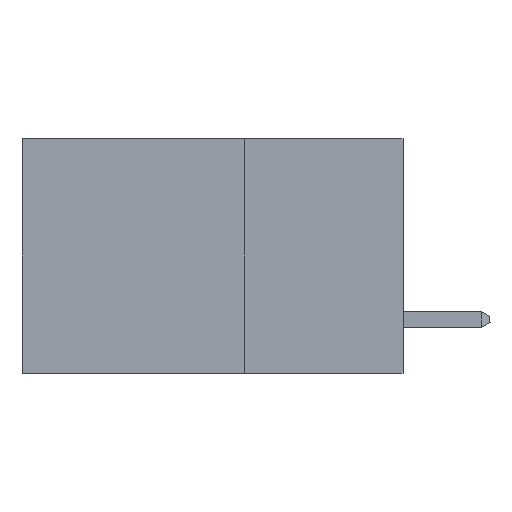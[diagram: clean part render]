
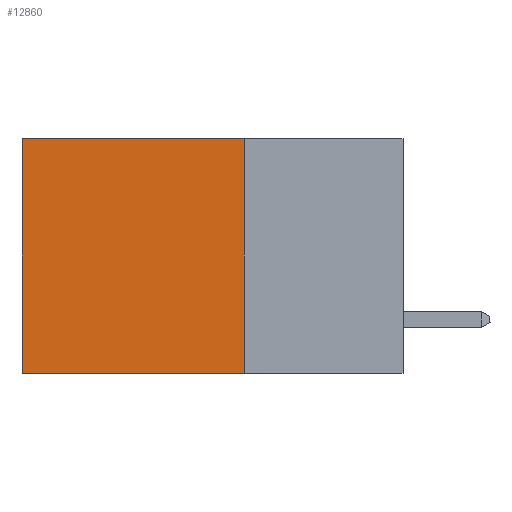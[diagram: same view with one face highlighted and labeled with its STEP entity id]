
A CAD part, left-side view. The second image highlights one B-rep face of the part: STEP entity #12860.
In plain terms, the highlighted planar face has unit normal (-1, 0, 0).
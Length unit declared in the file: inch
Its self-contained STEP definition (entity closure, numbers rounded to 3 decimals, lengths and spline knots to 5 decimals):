
#571 = VECTOR ( 'NONE', #19544, 39.37008 ) ;
#1139 = EDGE_LOOP ( 'NONE', ( #31832, #31684, #18330, #26916 ) ) ;
#1564 = CARTESIAN_POINT ( 'NONE',  ( 0.2875, 0.25, 0. ) ) ;
#1899 = CARTESIAN_POINT ( 'NONE',  ( 0.2875, 0.25, 0. ) ) ;
#2205 = CARTESIAN_POINT ( 'NONE',  ( 0.2875, 0.25, -0.37 ) ) ;
#3318 = DIRECTION ( 'NONE',  ( 0., 0., -1. ) ) ;
#3940 = CARTESIAN_POINT ( 'NONE',  ( 0.2875, 0.6, -0.37 ) ) ;
#4380 = LINE ( 'NONE', #1899, #24068 ) ;
#5832 = CARTESIAN_POINT ( 'NONE',  ( 0.2875, 0.6, 0. ) ) ;
#6565 = VECTOR ( 'NONE', #7022, 39.37008 ) ;
#7022 = DIRECTION ( 'NONE',  ( 0., 0., -1. ) ) ;
#10227 = EDGE_CURVE ( 'NONE', #18387, #23535, #30323, .T. ) ;
#10853 = EDGE_CURVE ( 'NONE', #13959, #18387, #22733, .T. ) ;
#12860 = ADVANCED_FACE ( 'NONE', ( #23487 ), #25109, .F. ) ;
#13561 = CARTESIAN_POINT ( 'NONE',  ( 0.2875, 0.25, 0. ) ) ;
#13959 = VERTEX_POINT ( 'NONE', #13561 ) ;
#14165 = AXIS2_PLACEMENT_3D ( 'NONE', #30395, #30273, #3318 ) ;
#14947 = EDGE_CURVE ( 'NONE', #31465, #23535, #27506, .T. ) ;
#17401 = DIRECTION ( 'NONE',  ( 0., 0., -1. ) ) ;
#17720 = EDGE_CURVE ( 'NONE', #13959, #31465, #4380, .T. ) ;
#18330 = ORIENTED_EDGE ( 'NONE', *, *, #10853, .F. ) ;
#18387 = VERTEX_POINT ( 'NONE', #2205 ) ;
#19544 = DIRECTION ( 'NONE',  ( 0., 1., 0. ) ) ;
#20146 = CARTESIAN_POINT ( 'NONE',  ( 0.2875, 0.6, 0. ) ) ;
#20505 = DIRECTION ( 'NONE',  ( 0., 1., 0. ) ) ;
#22733 = LINE ( 'NONE', #1564, #27770 ) ;
#23487 = FACE_OUTER_BOUND ( 'NONE', #1139, .T. ) ;
#23535 = VERTEX_POINT ( 'NONE', #3940 ) ;
#24068 = VECTOR ( 'NONE', #20505, 39.37008 ) ;
#25109 = PLANE ( 'NONE',  #14165 ) ;
#26916 = ORIENTED_EDGE ( 'NONE', *, *, #17720, .T. ) ;
#27402 = CARTESIAN_POINT ( 'NONE',  ( 0.2875, 0.25, -0.37 ) ) ;
#27506 = LINE ( 'NONE', #20146, #6565 ) ;
#27770 = VECTOR ( 'NONE', #17401, 39.37008 ) ;
#30273 = DIRECTION ( 'NONE',  ( 1., 0., 0. ) ) ;
#30323 = LINE ( 'NONE', #27402, #571 ) ;
#30395 = CARTESIAN_POINT ( 'NONE',  ( 0.2875, 0.25, 0. ) ) ;
#31465 = VERTEX_POINT ( 'NONE', #5832 ) ;
#31684 = ORIENTED_EDGE ( 'NONE', *, *, #10227, .F. ) ;
#31832 = ORIENTED_EDGE ( 'NONE', *, *, #14947, .T. ) ;
